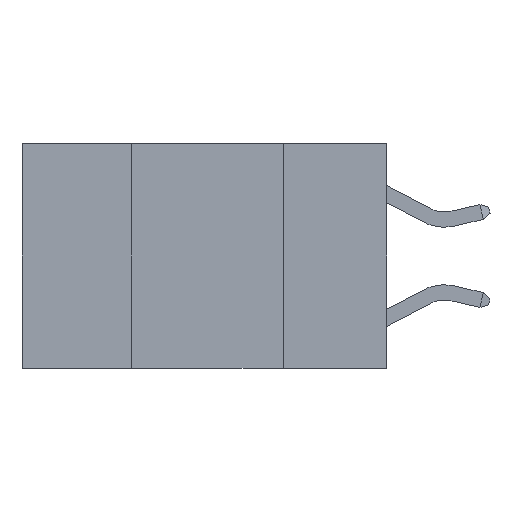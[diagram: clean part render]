
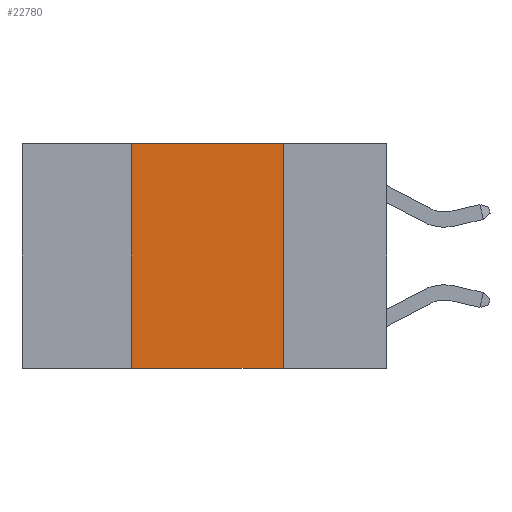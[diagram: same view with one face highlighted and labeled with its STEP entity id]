
A CAD part, left-side view. The second image highlights one B-rep face of the part: STEP entity #22780.
In plain terms, the highlighted planar face has unit normal (-1, 0, 0).
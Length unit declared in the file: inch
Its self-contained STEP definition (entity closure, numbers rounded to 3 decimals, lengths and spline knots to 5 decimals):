
#465 = PLANE ( 'NONE',  #19902 ) ;
#1415 = VERTEX_POINT ( 'NONE', #8298 ) ;
#1483 = EDGE_CURVE ( 'NONE', #8616, #7719, #6711, .T. ) ;
#1807 = VECTOR ( 'NONE', #4175, 39.37008 ) ;
#2423 = CARTESIAN_POINT ( 'NONE',  ( 0., 0.6, 0. ) ) ;
#2906 = EDGE_LOOP ( 'NONE', ( #13558, #8099, #19782, #14497 ) ) ;
#3054 = CARTESIAN_POINT ( 'NONE',  ( 0., 0.17, -0.37 ) ) ;
#4175 = DIRECTION ( 'NONE',  ( 0., -1., 0. ) ) ;
#4856 = CARTESIAN_POINT ( 'NONE',  ( 0., 0.6, -0.37 ) ) ;
#5166 = CARTESIAN_POINT ( 'NONE',  ( 0., 0.42, -0.37 ) ) ;
#5996 = DIRECTION ( 'NONE',  ( 0., 0., 1. ) ) ;
#6131 = EDGE_CURVE ( 'NONE', #23219, #7719, #8682, .T. ) ;
#6711 = LINE ( 'NONE', #4856, #1807 ) ;
#7666 = VECTOR ( 'NONE', #5996, 39.37008 ) ;
#7719 = VERTEX_POINT ( 'NONE', #3054 ) ;
#8099 = ORIENTED_EDGE ( 'NONE', *, *, #16793, .F. ) ;
#8298 = CARTESIAN_POINT ( 'NONE',  ( 0., 0.42, 0. ) ) ;
#8616 = VERTEX_POINT ( 'NONE', #5166 ) ;
#8682 = LINE ( 'NONE', #9591, #21968 ) ;
#9591 = CARTESIAN_POINT ( 'NONE',  ( 0., 0.17, 0. ) ) ;
#9749 = CARTESIAN_POINT ( 'NONE',  ( 0., 0.6, 0. ) ) ;
#11575 = DIRECTION ( 'NONE',  ( 1., 0., 0. ) ) ;
#11603 = DIRECTION ( 'NONE',  ( 0., -1., 0. ) ) ;
#13407 = LINE ( 'NONE', #9749, #22359 ) ;
#13558 = ORIENTED_EDGE ( 'NONE', *, *, #6131, .F. ) ;
#14497 = ORIENTED_EDGE ( 'NONE', *, *, #1483, .T. ) ;
#16793 = EDGE_CURVE ( 'NONE', #1415, #23219, #13407, .T. ) ;
#17062 = DIRECTION ( 'NONE',  ( 0., 0., -1. ) ) ;
#17370 = LINE ( 'NONE', #22227, #7666 ) ;
#19552 = EDGE_CURVE ( 'NONE', #8616, #1415, #17370, .T. ) ;
#19782 = ORIENTED_EDGE ( 'NONE', *, *, #19552, .F. ) ;
#19902 = AXIS2_PLACEMENT_3D ( 'NONE', #2423, #11575, #17062 ) ;
#20444 = DIRECTION ( 'NONE',  ( 0., 0., -1. ) ) ;
#21693 = FACE_OUTER_BOUND ( 'NONE', #2906, .T. ) ;
#21809 = CARTESIAN_POINT ( 'NONE',  ( 0., 0.17, 0. ) ) ;
#21968 = VECTOR ( 'NONE', #20444, 39.37008 ) ;
#22227 = CARTESIAN_POINT ( 'NONE',  ( 0., 0.42, 0. ) ) ;
#22359 = VECTOR ( 'NONE', #11603, 39.37008 ) ;
#22780 = ADVANCED_FACE ( 'NONE', ( #21693 ), #465, .F. ) ;
#23219 = VERTEX_POINT ( 'NONE', #21809 ) ;
